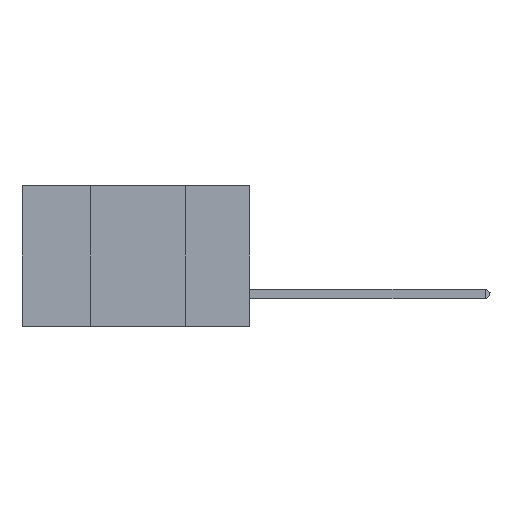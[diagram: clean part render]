
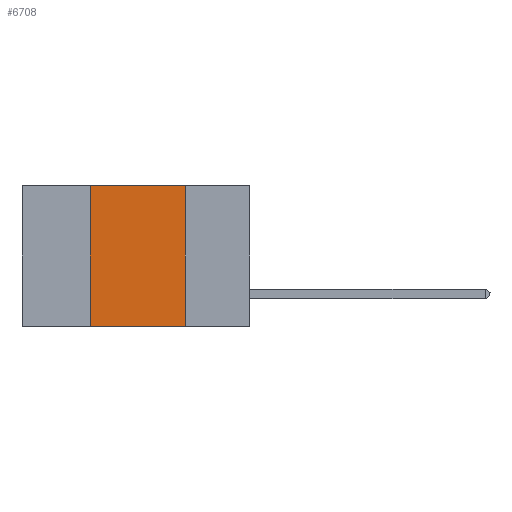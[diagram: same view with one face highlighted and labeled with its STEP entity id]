
A CAD part, left-side view. The second image highlights one B-rep face of the part: STEP entity #6708.
In plain terms, the highlighted planar face has unit normal (-1, 0, 0).
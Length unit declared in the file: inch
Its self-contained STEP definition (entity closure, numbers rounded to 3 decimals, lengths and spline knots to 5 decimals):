
#1181 = ORIENTED_EDGE ( 'NONE', *, *, #38254, .F. ) ;
#1484 = CARTESIAN_POINT ( 'NONE',  ( 0., 0.42, 0. ) ) ;
#3923 = VECTOR ( 'NONE', #42327, 39.37008 ) ;
#4199 = VECTOR ( 'NONE', #8055, 39.37008 ) ;
#4478 = ORIENTED_EDGE ( 'NONE', *, *, #12686, .F. ) ;
#6708 = ADVANCED_FACE ( 'NONE', ( #20615 ), #15627, .F. ) ;
#8055 = DIRECTION ( 'NONE',  ( 0., 0., -1. ) ) ;
#11252 = VECTOR ( 'NONE', #36064, 39.37008 ) ;
#11912 = EDGE_LOOP ( 'NONE', ( #4478, #1181, #41990, #15554 ) ) ;
#12230 = CARTESIAN_POINT ( 'NONE',  ( 0., 0.6, -0.37 ) ) ;
#12686 = EDGE_CURVE ( 'NONE', #13244, #22450, #22120, .T. ) ;
#13244 = VERTEX_POINT ( 'NONE', #24894 ) ;
#15182 = CARTESIAN_POINT ( 'NONE',  ( 0., 0.42, 0. ) ) ;
#15554 = ORIENTED_EDGE ( 'NONE', *, *, #27880, .T. ) ;
#15627 = PLANE ( 'NONE',  #27056 ) ;
#16822 = DIRECTION ( 'NONE',  ( 0., 0., -1. ) ) ;
#17478 = VERTEX_POINT ( 'NONE', #39734 ) ;
#18529 = CARTESIAN_POINT ( 'NONE',  ( 0., 0.6, 0. ) ) ;
#18590 = CARTESIAN_POINT ( 'NONE',  ( 0., 0.6, 0. ) ) ;
#19310 = DIRECTION ( 'NONE',  ( 1., 0., 0. ) ) ;
#20615 = FACE_OUTER_BOUND ( 'NONE', #11912, .T. ) ;
#21556 = CARTESIAN_POINT ( 'NONE',  ( 0., 0.17, 0. ) ) ;
#21648 = EDGE_CURVE ( 'NONE', #17478, #42296, #38645, .T. ) ;
#22120 = LINE ( 'NONE', #21556, #4199 ) ;
#22450 = VERTEX_POINT ( 'NONE', #30806 ) ;
#24894 = CARTESIAN_POINT ( 'NONE',  ( 0., 0.17, 0. ) ) ;
#25366 = DIRECTION ( 'NONE',  ( 0., -1., 0. ) ) ;
#27056 = AXIS2_PLACEMENT_3D ( 'NONE', #18529, #19310, #16822 ) ;
#27880 = EDGE_CURVE ( 'NONE', #17478, #22450, #39638, .T. ) ;
#30806 = CARTESIAN_POINT ( 'NONE',  ( 0., 0.17, -0.37 ) ) ;
#36064 = DIRECTION ( 'NONE',  ( 0., -1., 0. ) ) ;
#38237 = VECTOR ( 'NONE', #25366, 39.37008 ) ;
#38254 = EDGE_CURVE ( 'NONE', #42296, #13244, #38808, .T. ) ;
#38645 = LINE ( 'NONE', #1484, #3923 ) ;
#38808 = LINE ( 'NONE', #18590, #38237 ) ;
#39638 = LINE ( 'NONE', #12230, #11252 ) ;
#39734 = CARTESIAN_POINT ( 'NONE',  ( 0., 0.42, -0.37 ) ) ;
#41990 = ORIENTED_EDGE ( 'NONE', *, *, #21648, .F. ) ;
#42296 = VERTEX_POINT ( 'NONE', #15182 ) ;
#42327 = DIRECTION ( 'NONE',  ( 0., 0., 1. ) ) ;
